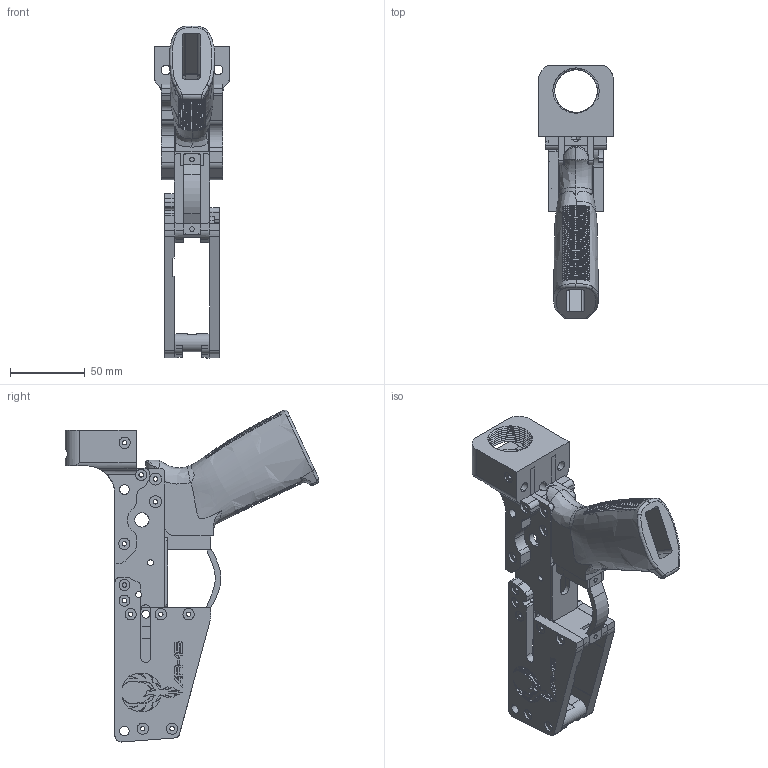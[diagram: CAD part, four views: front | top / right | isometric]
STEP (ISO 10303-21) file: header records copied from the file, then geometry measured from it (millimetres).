
FILE_DESCRIPTION (( 'STEP AP214' ), '1' );
FILE_NAME ('Firebolt_5.56_UBolt.STEP', '2020-12-05T18:46:22', ( '' ), ( '' ), 'SwSTEP 2.0', 'SolidWorks 2020', '' );
FILE_SCHEMA (( 'AUTOMOTIVE_DESIGN' ));
Length unit declared in the file: millimetre
Products named in the file (12): Firebolt_5.56_UBolt; Firebolt_Fire_Control_Well_Bottom; Firebolt_Mag_Well_Left; Firebolt_UBolt_Pistol_Grip; Firebolt_UBolt_Side_Right; Firebolt_UBolt_Grip_Part; Firebolt_UBolt_Buffer_Tower; Firebolt_UBolt_Side_Left; Firebolt_Trigger_Guard; Firebolt_Mag_Well_Rear; Firebolt_Mag_Well_Right; Firebolt_Mag_Well_Front
Assembly tree (11 placements, depth 2):
  Firebolt_5.56_UBolt
    Firebolt_UBolt_Buffer_Tower
    Firebolt_UBolt_Side_Left
    Firebolt_UBolt_Side_Right
    Firebolt_UBolt_Grip_Part
    Firebolt_UBolt_Pistol_Grip
    Firebolt_Fire_Control_Well_Bottom
    Firebolt_Trigger_Guard
    Firebolt_Mag_Well_Rear
    Firebolt_Mag_Well_Left
    Firebolt_Mag_Well_Front
    Firebolt_Mag_Well_Right
Bounding box: 50 x 170.14 x 222.59 mm (x, y, z)
Volume: 262258.2 mm3; surface area: 118608.4 mm2
Topology: 11 solids, 11 shells, 2129 faces, 6481 edges, 4412 vertices
Faces by surface type: plane 1456, cylinder 405, bspline 258, sphere 7, cone 3
Entity records: 138105 total; most frequent: CARTESIAN_POINT 82695, ORIENTED_EDGE 12958, DIRECTION 9208, EDGE_CURVE 6479, VERTEX_POINT 4412, VECTOR 4062, LINE 4062, AXIS2_PLACEMENT_3D 2573
